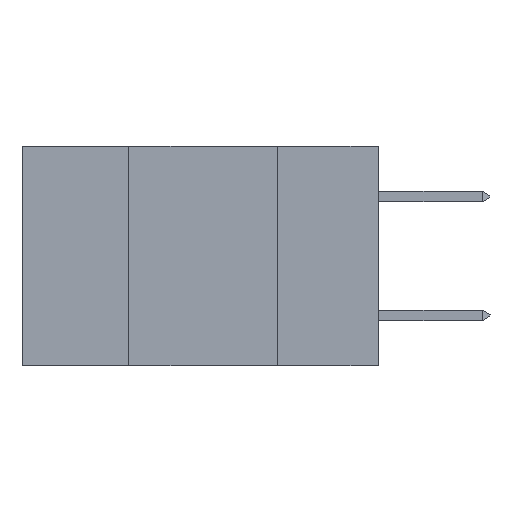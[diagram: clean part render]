
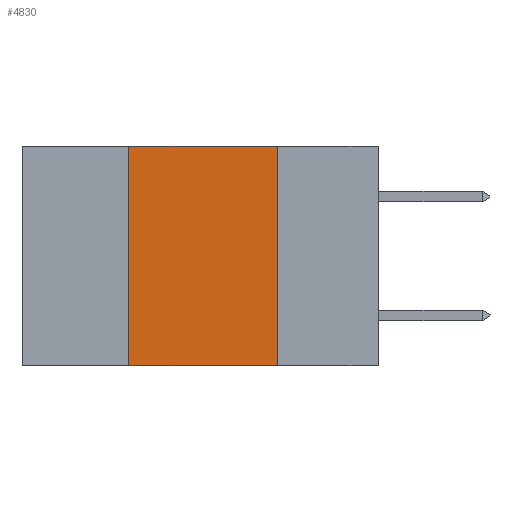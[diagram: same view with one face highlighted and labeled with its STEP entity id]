
A CAD part, left-side view. The second image highlights one B-rep face of the part: STEP entity #4830.
In plain terms, the highlighted planar face has unit normal (-1, 0, 0).
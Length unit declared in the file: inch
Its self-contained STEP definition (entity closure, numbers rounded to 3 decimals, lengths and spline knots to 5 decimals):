
#1191 = LINE ( 'NONE', #1596, #19038 ) ;
#1596 = CARTESIAN_POINT ( 'NONE',  ( 0., 0.42, 0. ) ) ;
#2225 = ORIENTED_EDGE ( 'NONE', *, *, #3458, .T. ) ;
#2498 = EDGE_LOOP ( 'NONE', ( #9197, #8699, #6189, #2225 ) ) ;
#2669 = CARTESIAN_POINT ( 'NONE',  ( 0., 0.42, -0.37 ) ) ;
#3458 = EDGE_CURVE ( 'NONE', #13976, #20673, #14812, .T. ) ;
#4830 = ADVANCED_FACE ( 'NONE', ( #7211 ), #17210, .F. ) ;
#5249 = DIRECTION ( 'NONE',  ( 0., 0., 1. ) ) ;
#6189 = ORIENTED_EDGE ( 'NONE', *, *, #20507, .F. ) ;
#6897 = CARTESIAN_POINT ( 'NONE',  ( 0., 0.42, 0. ) ) ;
#7211 = FACE_OUTER_BOUND ( 'NONE', #2498, .T. ) ;
#7635 = CARTESIAN_POINT ( 'NONE',  ( 0., 0.6, -0.37 ) ) ;
#8699 = ORIENTED_EDGE ( 'NONE', *, *, #9892, .F. ) ;
#9197 = ORIENTED_EDGE ( 'NONE', *, *, #14883, .F. ) ;
#9892 = EDGE_CURVE ( 'NONE', #14632, #18585, #17315, .T. ) ;
#9982 = VECTOR ( 'NONE', #18318, 39.37008 ) ;
#11142 = CARTESIAN_POINT ( 'NONE',  ( 0., 0.6, 0. ) ) ;
#11287 = DIRECTION ( 'NONE',  ( 0., -1., 0. ) ) ;
#12999 = AXIS2_PLACEMENT_3D ( 'NONE', #16987, #19738, #17216 ) ;
#13288 = CARTESIAN_POINT ( 'NONE',  ( 0., 0.17, -0.37 ) ) ;
#13976 = VERTEX_POINT ( 'NONE', #2669 ) ;
#14274 = CARTESIAN_POINT ( 'NONE',  ( 0., 0.17, 0. ) ) ;
#14632 = VERTEX_POINT ( 'NONE', #6897 ) ;
#14812 = LINE ( 'NONE', #7635, #9982 ) ;
#14883 = EDGE_CURVE ( 'NONE', #18585, #20673, #22179, .T. ) ;
#16172 = CARTESIAN_POINT ( 'NONE',  ( 0., 0.17, 0. ) ) ;
#16987 = CARTESIAN_POINT ( 'NONE',  ( 0., 0.6, 0. ) ) ;
#17210 = PLANE ( 'NONE',  #12999 ) ;
#17216 = DIRECTION ( 'NONE',  ( 0., 0., -1. ) ) ;
#17315 = LINE ( 'NONE', #11142, #20560 ) ;
#18318 = DIRECTION ( 'NONE',  ( 0., -1., 0. ) ) ;
#18585 = VERTEX_POINT ( 'NONE', #16172 ) ;
#18653 = VECTOR ( 'NONE', #21542, 39.37008 ) ;
#19038 = VECTOR ( 'NONE', #5249, 39.37008 ) ;
#19738 = DIRECTION ( 'NONE',  ( 1., 0., 0. ) ) ;
#20507 = EDGE_CURVE ( 'NONE', #13976, #14632, #1191, .T. ) ;
#20560 = VECTOR ( 'NONE', #11287, 39.37008 ) ;
#20673 = VERTEX_POINT ( 'NONE', #13288 ) ;
#21542 = DIRECTION ( 'NONE',  ( 0., 0., -1. ) ) ;
#22179 = LINE ( 'NONE', #14274, #18653 ) ;
